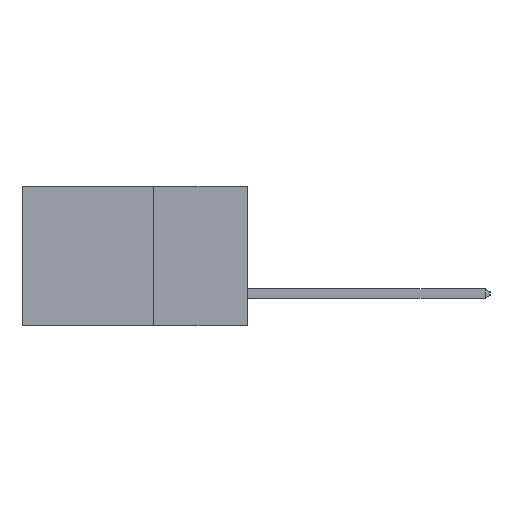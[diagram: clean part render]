
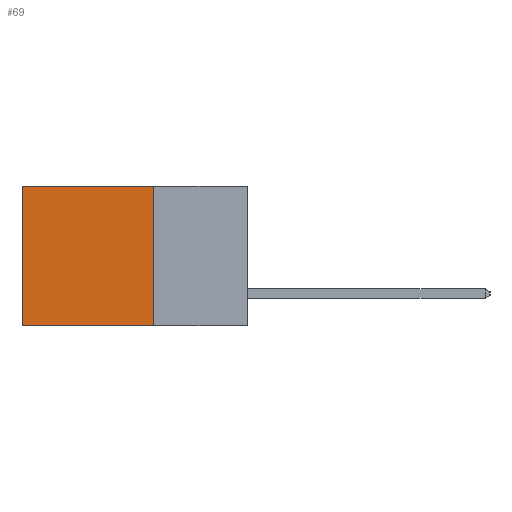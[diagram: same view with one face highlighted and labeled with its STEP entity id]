
A CAD part, left-side view. The second image highlights one B-rep face of the part: STEP entity #69.
In plain terms, the highlighted planar face has unit normal (-1, 0, 0).
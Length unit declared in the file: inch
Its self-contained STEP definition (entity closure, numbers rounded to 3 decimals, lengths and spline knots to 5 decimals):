
#61 = CARTESIAN_POINT ( 'NONE',  ( 0.2615, 0.6, -0.37 ) ) ;
#69 = ADVANCED_FACE ( 'NONE', ( #16086 ), #8163, .F. ) ;
#319 = EDGE_CURVE ( 'NONE', #16031, #12513, #1460, .T. ) ;
#555 = DIRECTION ( 'NONE',  ( 0., 0., -1. ) ) ;
#798 = AXIS2_PLACEMENT_3D ( 'NONE', #7169, #13468, #13938 ) ;
#1460 = LINE ( 'NONE', #9674, #16285 ) ;
#2313 = LINE ( 'NONE', #9724, #8878 ) ;
#2355 = CARTESIAN_POINT ( 'NONE',  ( 0.2615, 0.25, -0.37 ) ) ;
#2399 = ORIENTED_EDGE ( 'NONE', *, *, #12205, .F. ) ;
#2970 = CARTESIAN_POINT ( 'NONE',  ( 0.2615, 0.25, -0.37 ) ) ;
#3347 = CARTESIAN_POINT ( 'NONE',  ( 0.2615, 0.6, 0. ) ) ;
#3406 = VECTOR ( 'NONE', #10218, 39.37008 ) ;
#4251 = CARTESIAN_POINT ( 'NONE',  ( 0.2615, 0.25, 0. ) ) ;
#5410 = EDGE_LOOP ( 'NONE', ( #11083, #2399, #5896, #5516 ) ) ;
#5516 = ORIENTED_EDGE ( 'NONE', *, *, #9241, .T. ) ;
#5553 = DIRECTION ( 'NONE',  ( 0., 1., 0. ) ) ;
#5896 = ORIENTED_EDGE ( 'NONE', *, *, #319, .F. ) ;
#6331 = CARTESIAN_POINT ( 'NONE',  ( 0.2615, 0.25, 0. ) ) ;
#6851 = LINE ( 'NONE', #2355, #3406 ) ;
#7169 = CARTESIAN_POINT ( 'NONE',  ( 0.2615, 0.25, -0.37 ) ) ;
#8163 = PLANE ( 'NONE',  #798 ) ;
#8668 = LINE ( 'NONE', #4251, #15282 ) ;
#8878 = VECTOR ( 'NONE', #555, 39.37008 ) ;
#9016 = EDGE_CURVE ( 'NONE', #9455, #10419, #2313, .T. ) ;
#9241 = EDGE_CURVE ( 'NONE', #16031, #9455, #8668, .T. ) ;
#9455 = VERTEX_POINT ( 'NONE', #3347 ) ;
#9674 = CARTESIAN_POINT ( 'NONE',  ( 0.2615, 0.25, -0.37 ) ) ;
#9724 = CARTESIAN_POINT ( 'NONE',  ( 0.2615, 0.6, -0.37 ) ) ;
#10218 = DIRECTION ( 'NONE',  ( 0., 1., 0. ) ) ;
#10419 = VERTEX_POINT ( 'NONE', #61 ) ;
#11006 = DIRECTION ( 'NONE',  ( 0., 0., -1. ) ) ;
#11083 = ORIENTED_EDGE ( 'NONE', *, *, #9016, .T. ) ;
#12205 = EDGE_CURVE ( 'NONE', #12513, #10419, #6851, .T. ) ;
#12513 = VERTEX_POINT ( 'NONE', #2970 ) ;
#13468 = DIRECTION ( 'NONE',  ( 1., 0., 0. ) ) ;
#13938 = DIRECTION ( 'NONE',  ( 0., 0., -1. ) ) ;
#15282 = VECTOR ( 'NONE', #5553, 39.37008 ) ;
#16031 = VERTEX_POINT ( 'NONE', #6331 ) ;
#16086 = FACE_OUTER_BOUND ( 'NONE', #5410, .T. ) ;
#16285 = VECTOR ( 'NONE', #11006, 39.37008 ) ;
